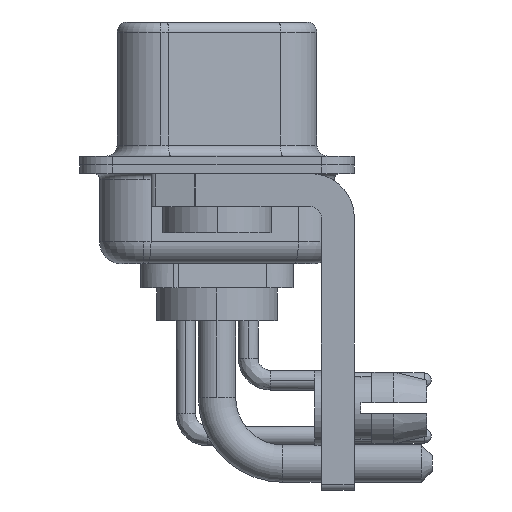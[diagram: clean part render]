
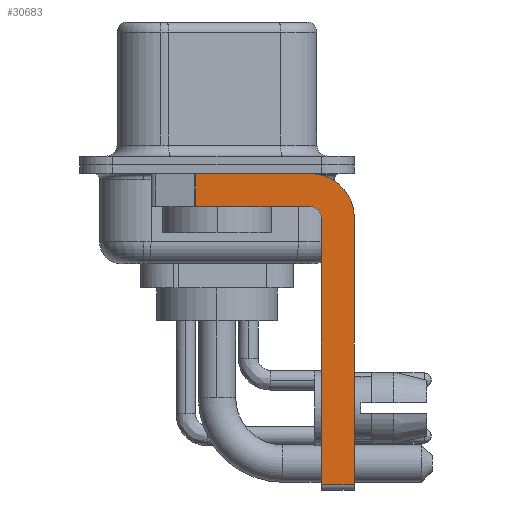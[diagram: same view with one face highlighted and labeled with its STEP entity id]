
A CAD part, left-side view. The second image highlights one B-rep face of the part: STEP entity #30683.
In plain terms, the highlighted planar face has unit normal (-1, 0, 0).
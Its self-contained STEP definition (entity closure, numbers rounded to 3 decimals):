
#273 = CARTESIAN_POINT ( 'NONE',  ( -2.9, -6.25, -2.4 ) ) ;
#901 = CARTESIAN_POINT ( 'NONE',  ( -2.9, -6.25, -14.55 ) ) ;
#918 = VECTOR ( 'NONE', #2720, 1000. ) ;
#1136 = ORIENTED_EDGE ( 'NONE', *, *, #18396, .F. ) ;
#2298 = VECTOR ( 'NONE', #3950, 1000. ) ;
#2720 = DIRECTION ( 'NONE',  ( 0., -1., 0. ) ) ;
#2721 = VECTOR ( 'NONE', #18991, 1000. ) ;
#2831 = VERTEX_POINT ( 'NONE', #12665 ) ;
#3400 = LINE ( 'NONE', #22243, #23897 ) ;
#3950 = DIRECTION ( 'NONE',  ( 0., 0., -1. ) ) ;
#3956 = CARTESIAN_POINT ( 'NONE',  ( -2.9, -4.75, -2.4 ) ) ;
#3965 = EDGE_LOOP ( 'NONE', ( #6030, #5705, #1136, #5245, #22674, #29693, #15622, #15240 ) ) ;
#4601 = VERTEX_POINT ( 'NONE', #27195 ) ;
#5245 = ORIENTED_EDGE ( 'NONE', *, *, #14791, .F. ) ;
#5705 = ORIENTED_EDGE ( 'NONE', *, *, #20409, .T. ) ;
#5950 = AXIS2_PLACEMENT_3D ( 'NONE', #19432, #22102, #17391 ) ;
#6030 = ORIENTED_EDGE ( 'NONE', *, *, #22248, .F. ) ;
#6059 = CARTESIAN_POINT ( 'NONE',  ( -2.9, -4.25, -14.55 ) ) ;
#7950 = AXIS2_PLACEMENT_3D ( 'NONE', #18724, #11222, #25820 ) ;
#8368 = DIRECTION ( 'NONE',  ( 1., 0., 0. ) ) ;
#8762 = VERTEX_POINT ( 'NONE', #3956 ) ;
#8842 = CARTESIAN_POINT ( 'NONE',  ( -2.9, -6.25, -2.4 ) ) ;
#8977 = CIRCLE ( 'NONE', #5950, 0.5 ) ;
#9484 = DIRECTION ( 'NONE',  ( 0., 0., 1. ) ) ;
#11103 = VERTEX_POINT ( 'NONE', #901 ) ;
#11222 = DIRECTION ( 'NONE',  ( 1., 0., 0. ) ) ;
#11904 = VERTEX_POINT ( 'NONE', #28528 ) ;
#12665 = CARTESIAN_POINT ( 'NONE',  ( -2.9, -4.25, -1.9 ) ) ;
#13038 = VECTOR ( 'NONE', #15663, 1000. ) ;
#13370 = AXIS2_PLACEMENT_3D ( 'NONE', #14566, #8368, #30093 ) ;
#14152 = LINE ( 'NONE', #22393, #2721 ) ;
#14566 = CARTESIAN_POINT ( 'NONE',  ( -2.9, -4.25, -2.4 ) ) ;
#14791 = EDGE_CURVE ( 'NONE', #8762, #2831, #8977, .T. ) ;
#15240 = ORIENTED_EDGE ( 'NONE', *, *, #22048, .F. ) ;
#15505 = VERTEX_POINT ( 'NONE', #25799 ) ;
#15622 = ORIENTED_EDGE ( 'NONE', *, *, #30883, .F. ) ;
#15663 = DIRECTION ( 'NONE',  ( 0., -1., 0. ) ) ;
#15975 = VERTEX_POINT ( 'NONE', #273 ) ;
#16906 = FACE_OUTER_BOUND ( 'NONE', #3965, .T. ) ;
#17036 = LINE ( 'NONE', #24249, #918 ) ;
#17391 = DIRECTION ( 'NONE',  ( 0., 0., 1. ) ) ;
#18396 = EDGE_CURVE ( 'NONE', #2831, #15505, #14152, .T. ) ;
#18558 = LINE ( 'NONE', #8842, #2298 ) ;
#18724 = CARTESIAN_POINT ( 'NONE',  ( -2.9, -4.25, -2.4 ) ) ;
#18727 = LINE ( 'NONE', #20931, #27901 ) ;
#18991 = DIRECTION ( 'NONE',  ( 0., 1., 0. ) ) ;
#19127 = EDGE_CURVE ( 'NONE', #11904, #8762, #18727, .T. ) ;
#19432 = CARTESIAN_POINT ( 'NONE',  ( -2.9, -4.25, -2.4 ) ) ;
#19891 = DIRECTION ( 'NONE',  ( 0., 0., -1. ) ) ;
#19952 = CARTESIAN_POINT ( 'NONE',  ( -2.9, 0.978, -0.4 ) ) ;
#20409 = EDGE_CURVE ( 'NONE', #24134, #15505, #3400, .T. ) ;
#20931 = CARTESIAN_POINT ( 'NONE',  ( -2.9, -4.75, -14.8 ) ) ;
#22048 = EDGE_CURVE ( 'NONE', #4601, #15975, #23514, .T. ) ;
#22102 = DIRECTION ( 'NONE',  ( -1., 0., 0. ) ) ;
#22243 = CARTESIAN_POINT ( 'NONE',  ( -2.9, 0.978, -1.9 ) ) ;
#22248 = EDGE_CURVE ( 'NONE', #24134, #4601, #17036, .T. ) ;
#22393 = CARTESIAN_POINT ( 'NONE',  ( -2.9, -4.25, -1.9 ) ) ;
#22674 = ORIENTED_EDGE ( 'NONE', *, *, #19127, .F. ) ;
#23029 = LINE ( 'NONE', #6059, #13038 ) ;
#23121 = EDGE_CURVE ( 'NONE', #11904, #11103, #23029, .T. ) ;
#23514 = CIRCLE ( 'NONE', #7950, 2. ) ;
#23897 = VECTOR ( 'NONE', #19891, 1000. ) ;
#24134 = VERTEX_POINT ( 'NONE', #19952 ) ;
#24249 = CARTESIAN_POINT ( 'NONE',  ( -2.9, 3., -0.4 ) ) ;
#25799 = CARTESIAN_POINT ( 'NONE',  ( -2.9, 0.978, -1.9 ) ) ;
#25820 = DIRECTION ( 'NONE',  ( 0., 0., -1. ) ) ;
#26507 = PLANE ( 'NONE',  #13370 ) ;
#27195 = CARTESIAN_POINT ( 'NONE',  ( -2.9, -4.25, -0.4 ) ) ;
#27901 = VECTOR ( 'NONE', #9484, 1000. ) ;
#28528 = CARTESIAN_POINT ( 'NONE',  ( -2.9, -4.75, -14.55 ) ) ;
#29693 = ORIENTED_EDGE ( 'NONE', *, *, #23121, .T. ) ;
#30093 = DIRECTION ( 'NONE',  ( 0., 0., -1. ) ) ;
#30683 = ADVANCED_FACE ( 'NONE', ( #16906 ), #26507, .F. ) ;
#30883 = EDGE_CURVE ( 'NONE', #15975, #11103, #18558, .T. ) ;
